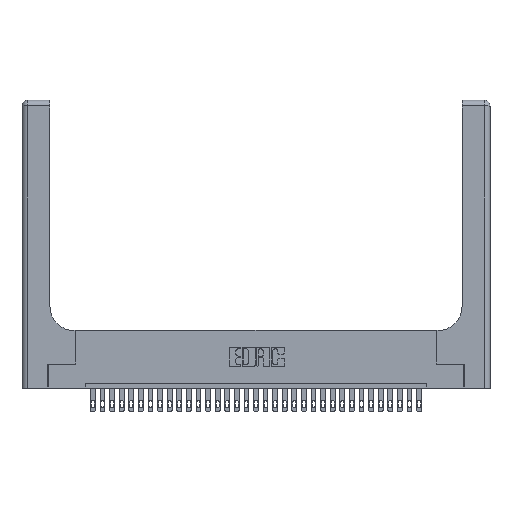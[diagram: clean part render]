
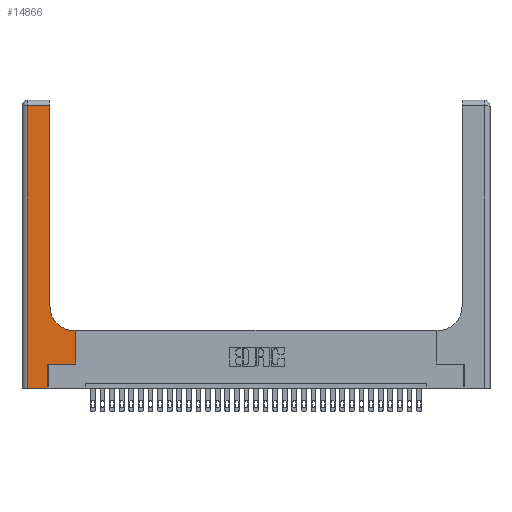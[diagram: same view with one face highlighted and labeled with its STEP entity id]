
A CAD part, top view. The second image highlights one B-rep face of the part: STEP entity #14866.
In plain terms, the highlighted planar face has unit normal (0, 0, 1).
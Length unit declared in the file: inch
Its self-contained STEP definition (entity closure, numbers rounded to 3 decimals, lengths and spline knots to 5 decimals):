
#18 = EDGE_CURVE ( 'NONE', #22363, #11315, #13458, .T. ) ;
#509 = EDGE_CURVE ( 'NONE', #2427, #17606, #13787, .T. ) ;
#528 = CARTESIAN_POINT ( 'NONE',  ( 0.5585, 0.6, 0.37 ) ) ;
#749 = DIRECTION ( 'NONE',  ( 1., 0., 0. ) ) ;
#845 = CIRCLE ( 'NONE', #21865, 0.25 ) ;
#884 = VECTOR ( 'NONE', #5573, 39.37008 ) ;
#1004 = CARTESIAN_POINT ( 'NONE',  ( 0.5585, 0.25, 0.37 ) ) ;
#1374 = EDGE_CURVE ( 'NONE', #15208, #22265, #3160, .T. ) ;
#1418 = VERTEX_POINT ( 'NONE', #8924 ) ;
#2427 = VERTEX_POINT ( 'NONE', #3510 ) ;
#3117 = FACE_OUTER_BOUND ( 'NONE', #28039, .T. ) ;
#3160 = LINE ( 'NONE', #24013, #21573 ) ;
#3510 = CARTESIAN_POINT ( 'NONE',  ( 0.2915, 0.85, 0.37 ) ) ;
#4056 = VECTOR ( 'NONE', #11927, 39.37008 ) ;
#4295 = LINE ( 'NONE', #20658, #5067 ) ;
#4866 = LINE ( 'NONE', #19040, #4056 ) ;
#5067 = VECTOR ( 'NONE', #30266, 39.37008 ) ;
#5078 = LINE ( 'NONE', #17365, #8626 ) ;
#5265 = PLANE ( 'NONE',  #30453 ) ;
#5475 = LINE ( 'NONE', #18039, #24680 ) ;
#5573 = DIRECTION ( 'NONE',  ( 0., 1., 0. ) ) ;
#6417 = ORIENTED_EDGE ( 'NONE', *, *, #29323, .T. ) ;
#7260 = DIRECTION ( 'NONE',  ( -1., 0., 0. ) ) ;
#7335 = EDGE_CURVE ( 'NONE', #17606, #22000, #5078, .T. ) ;
#7905 = CARTESIAN_POINT ( 'NONE',  ( 0.5415, 0.85, 0.37 ) ) ;
#8626 = VECTOR ( 'NONE', #7260, 39.37008 ) ;
#8757 = ORIENTED_EDGE ( 'NONE', *, *, #7335, .T. ) ;
#8924 = CARTESIAN_POINT ( 'NONE',  ( 0.5585, 0.25, 0.37 ) ) ;
#10015 = CARTESIAN_POINT ( 'NONE',  ( 0.06, 0., 0.37 ) ) ;
#10339 = DIRECTION ( 'NONE',  ( 0., 0., -1. ) ) ;
#10641 = CARTESIAN_POINT ( 'NONE',  ( 0.2915, 3., 0.37 ) ) ;
#10924 = CARTESIAN_POINT ( 'NONE',  ( 0.269, 0.25, 0.37 ) ) ;
#11315 = VERTEX_POINT ( 'NONE', #23444 ) ;
#11660 = DIRECTION ( 'NONE',  ( -1., 0., 0. ) ) ;
#11927 = DIRECTION ( 'NONE',  ( 0., 1., 0. ) ) ;
#13384 = DIRECTION ( 'NONE',  ( 1., 0., 0. ) ) ;
#13458 = LINE ( 'NONE', #30703, #27136 ) ;
#13787 = LINE ( 'NONE', #10641, #884 ) ;
#14866 = ADVANCED_FACE ( 'NONE', ( #3117 ), #5265, .F. ) ;
#15136 = VECTOR ( 'NONE', #26058, 39.37008 ) ;
#15208 = VERTEX_POINT ( 'NONE', #528 ) ;
#15571 = ORIENTED_EDGE ( 'NONE', *, *, #21157, .T. ) ;
#15666 = VERTEX_POINT ( 'NONE', #10924 ) ;
#17365 = CARTESIAN_POINT ( 'NONE',  ( 0., 2.94, 0.37 ) ) ;
#17606 = VERTEX_POINT ( 'NONE', #18910 ) ;
#17816 = ORIENTED_EDGE ( 'NONE', *, *, #29375, .T. ) ;
#18039 = CARTESIAN_POINT ( 'NONE',  ( 0.06, 3., 0.37 ) ) ;
#18910 = CARTESIAN_POINT ( 'NONE',  ( 0.2915, 2.94, 0.37 ) ) ;
#19040 = CARTESIAN_POINT ( 'NONE',  ( 0.269, 0., 0.37 ) ) ;
#19972 = CARTESIAN_POINT ( 'NONE',  ( 0.5415, 0.6, 0.37 ) ) ;
#20658 = CARTESIAN_POINT ( 'NONE',  ( 0.269, 0.25, 0.37 ) ) ;
#21157 = EDGE_CURVE ( 'NONE', #1418, #15208, #31561, .T. ) ;
#21573 = VECTOR ( 'NONE', #11660, 39.37008 ) ;
#21865 = AXIS2_PLACEMENT_3D ( 'NONE', #7905, #28129, #13384 ) ;
#21897 = ORIENTED_EDGE ( 'NONE', *, *, #24737, .T. ) ;
#22000 = VERTEX_POINT ( 'NONE', #31198 ) ;
#22265 = VERTEX_POINT ( 'NONE', #19972 ) ;
#22294 = ORIENTED_EDGE ( 'NONE', *, *, #23286, .T. ) ;
#22363 = VERTEX_POINT ( 'NONE', #10015 ) ;
#23286 = EDGE_CURVE ( 'NONE', #11315, #15666, #4866, .T. ) ;
#23444 = CARTESIAN_POINT ( 'NONE',  ( 0.269, 0., 0.37 ) ) ;
#24013 = CARTESIAN_POINT ( 'NONE',  ( 0.2915, 0.6, 0.37 ) ) ;
#24680 = VECTOR ( 'NONE', #30691, 39.37008 ) ;
#24737 = EDGE_CURVE ( 'NONE', #22265, #2427, #845, .T. ) ;
#25313 = CARTESIAN_POINT ( 'NONE',  ( 0., 3., 0.37 ) ) ;
#25838 = ORIENTED_EDGE ( 'NONE', *, *, #1374, .T. ) ;
#26058 = DIRECTION ( 'NONE',  ( 0., 1., 0. ) ) ;
#27136 = VECTOR ( 'NONE', #749, 39.37008 ) ;
#27798 = DIRECTION ( 'NONE',  ( -1., 0., 0. ) ) ;
#28039 = EDGE_LOOP ( 'NONE', ( #31988, #8757, #6417, #28610, #22294, #17816, #15571, #25838, #21897 ) ) ;
#28129 = DIRECTION ( 'NONE',  ( 0., 0., -1. ) ) ;
#28610 = ORIENTED_EDGE ( 'NONE', *, *, #18, .T. ) ;
#29323 = EDGE_CURVE ( 'NONE', #22000, #22363, #5475, .T. ) ;
#29375 = EDGE_CURVE ( 'NONE', #15666, #1418, #4295, .T. ) ;
#30266 = DIRECTION ( 'NONE',  ( 1., 0., 0. ) ) ;
#30453 = AXIS2_PLACEMENT_3D ( 'NONE', #25313, #10339, #27798 ) ;
#30691 = DIRECTION ( 'NONE',  ( 0., -1., 0. ) ) ;
#30703 = CARTESIAN_POINT ( 'NONE',  ( 0., 0., 0.37 ) ) ;
#31198 = CARTESIAN_POINT ( 'NONE',  ( 0.06, 2.94, 0.37 ) ) ;
#31561 = LINE ( 'NONE', #1004, #15136 ) ;
#31988 = ORIENTED_EDGE ( 'NONE', *, *, #509, .T. ) ;
